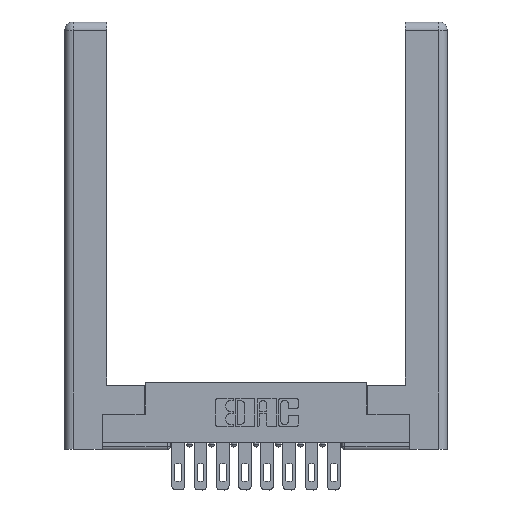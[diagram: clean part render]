
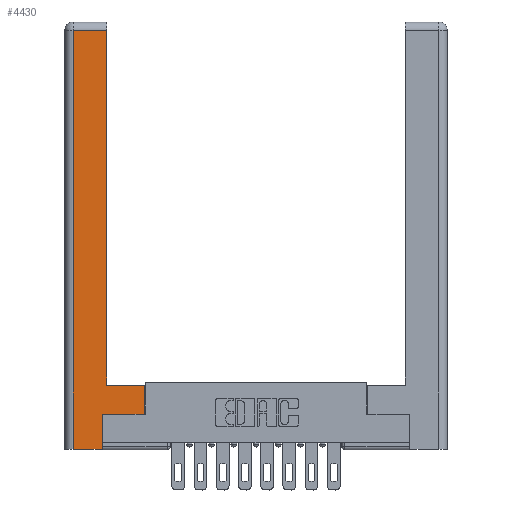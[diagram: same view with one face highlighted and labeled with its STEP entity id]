
A CAD part, top view. The second image highlights one B-rep face of the part: STEP entity #4430.
In plain terms, the highlighted planar face has unit normal (0, 0, 1).
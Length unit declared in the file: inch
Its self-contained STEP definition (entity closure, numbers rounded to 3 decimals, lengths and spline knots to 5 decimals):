
#186 = FACE_OUTER_BOUND ( 'NONE', #8757, .T. ) ;
#212 = DIRECTION ( 'NONE',  ( 0., 1., 0. ) ) ;
#252 = CARTESIAN_POINT ( 'NONE',  ( 0.265, 0.245, 0. ) ) ;
#420 = VECTOR ( 'NONE', #10739, 39.37008 ) ;
#593 = VERTEX_POINT ( 'NONE', #9906 ) ;
#1024 = VERTEX_POINT ( 'NONE', #7523 ) ;
#1460 = DIRECTION ( 'NONE',  ( 0., -1., 0. ) ) ;
#1492 = CARTESIAN_POINT ( 'NONE',  ( 0.565, 0.45, 0. ) ) ;
#1494 = ORIENTED_EDGE ( 'NONE', *, *, #10343, .T. ) ;
#1654 = VECTOR ( 'NONE', #6782, 39.37008 ) ;
#1965 = DIRECTION ( 'NONE',  ( -1., 0., 0. ) ) ;
#2482 = CARTESIAN_POINT ( 'NONE',  ( 0.265, 0.245, 0. ) ) ;
#2676 = VERTEX_POINT ( 'NONE', #10811 ) ;
#3039 = EDGE_CURVE ( 'NONE', #593, #1024, #3701, .T. ) ;
#3087 = DIRECTION ( 'NONE',  ( 1., 0., 0. ) ) ;
#3089 = VERTEX_POINT ( 'NONE', #6092 ) ;
#3150 = ORIENTED_EDGE ( 'NONE', *, *, #7372, .T. ) ;
#3421 = LINE ( 'NONE', #252, #7207 ) ;
#3577 = LINE ( 'NONE', #10787, #420 ) ;
#3701 = LINE ( 'NONE', #7057, #4202 ) ;
#3790 = DIRECTION ( 'NONE',  ( -1., 0., 0. ) ) ;
#3897 = EDGE_CURVE ( 'NONE', #3089, #8416, #6128, .T. ) ;
#4067 = VERTEX_POINT ( 'NONE', #2482 ) ;
#4142 = VECTOR ( 'NONE', #3790, 39.37008 ) ;
#4202 = VECTOR ( 'NONE', #6055, 39.37008 ) ;
#4238 = PLANE ( 'NONE',  #11466 ) ;
#4430 = ADVANCED_FACE ( 'NONE', ( #186 ), #4238, .F. ) ;
#4468 = LINE ( 'NONE', #1492, #1654 ) ;
#4824 = ORIENTED_EDGE ( 'NONE', *, *, #3897, .T. ) ;
#4943 = VERTEX_POINT ( 'NONE', #8390 ) ;
#5295 = CARTESIAN_POINT ( 'NONE',  ( 0.265, 0., 0. ) ) ;
#5551 = VECTOR ( 'NONE', #1460, 39.37008 ) ;
#5937 = LINE ( 'NONE', #6907, #4142 ) ;
#6055 = DIRECTION ( 'NONE',  ( 0., 1., 0. ) ) ;
#6092 = CARTESIAN_POINT ( 'NONE',  ( 0.0615, 0., 0. ) ) ;
#6128 = LINE ( 'NONE', #11761, #9254 ) ;
#6229 = LINE ( 'NONE', #12547, #7055 ) ;
#6517 = ORIENTED_EDGE ( 'NONE', *, *, #7354, .T. ) ;
#6782 = DIRECTION ( 'NONE',  ( 0., 1., 0. ) ) ;
#6907 = CARTESIAN_POINT ( 'NONE',  ( 0.295, 0.45, 0. ) ) ;
#7055 = VECTOR ( 'NONE', #3087, 39.37008 ) ;
#7057 = CARTESIAN_POINT ( 'NONE',  ( 0.295, 3., 0. ) ) ;
#7207 = VECTOR ( 'NONE', #212, 39.37008 ) ;
#7354 = EDGE_CURVE ( 'NONE', #4943, #12876, #4468, .T. ) ;
#7372 = EDGE_CURVE ( 'NONE', #12876, #593, #5937, .T. ) ;
#7523 = CARTESIAN_POINT ( 'NONE',  ( 0.295, 2.94, 0. ) ) ;
#7596 = DIRECTION ( 'NONE',  ( 1., 0., 0. ) ) ;
#7604 = ORIENTED_EDGE ( 'NONE', *, *, #13032, .T. ) ;
#7765 = CARTESIAN_POINT ( 'NONE',  ( 0.0615, 0., 0. ) ) ;
#7895 = ORIENTED_EDGE ( 'NONE', *, *, #3039, .T. ) ;
#8390 = CARTESIAN_POINT ( 'NONE',  ( 0.565, 0.245, 0. ) ) ;
#8416 = VERTEX_POINT ( 'NONE', #5295 ) ;
#8757 = EDGE_LOOP ( 'NONE', ( #7895, #1494, #13548, #4824, #13484, #7604, #6517, #3150 ) ) ;
#9041 = EDGE_CURVE ( 'NONE', #8416, #4067, #3421, .T. ) ;
#9210 = EDGE_CURVE ( 'NONE', #2676, #3089, #11167, .T. ) ;
#9254 = VECTOR ( 'NONE', #7596, 39.37008 ) ;
#9906 = CARTESIAN_POINT ( 'NONE',  ( 0.295, 0.45, 0. ) ) ;
#10343 = EDGE_CURVE ( 'NONE', #1024, #2676, #3577, .T. ) ;
#10739 = DIRECTION ( 'NONE',  ( -1., 0., 0. ) ) ;
#10787 = CARTESIAN_POINT ( 'NONE',  ( 0.0615, 2.94, 0. ) ) ;
#10811 = CARTESIAN_POINT ( 'NONE',  ( 0.0615, 2.94, 0. ) ) ;
#11167 = LINE ( 'NONE', #7765, #5551 ) ;
#11466 = AXIS2_PLACEMENT_3D ( 'NONE', #11605, #11649, #1965 ) ;
#11605 = CARTESIAN_POINT ( 'NONE',  ( 0., 0., 0. ) ) ;
#11649 = DIRECTION ( 'NONE',  ( 0., 0., -1. ) ) ;
#11761 = CARTESIAN_POINT ( 'NONE',  ( 0.265, 0., 0. ) ) ;
#12164 = CARTESIAN_POINT ( 'NONE',  ( 0.565, 0.45, 0. ) ) ;
#12547 = CARTESIAN_POINT ( 'NONE',  ( 0.565, 0.245, 0. ) ) ;
#12876 = VERTEX_POINT ( 'NONE', #12164 ) ;
#13032 = EDGE_CURVE ( 'NONE', #4067, #4943, #6229, .T. ) ;
#13484 = ORIENTED_EDGE ( 'NONE', *, *, #9041, .T. ) ;
#13548 = ORIENTED_EDGE ( 'NONE', *, *, #9210, .T. ) ;
